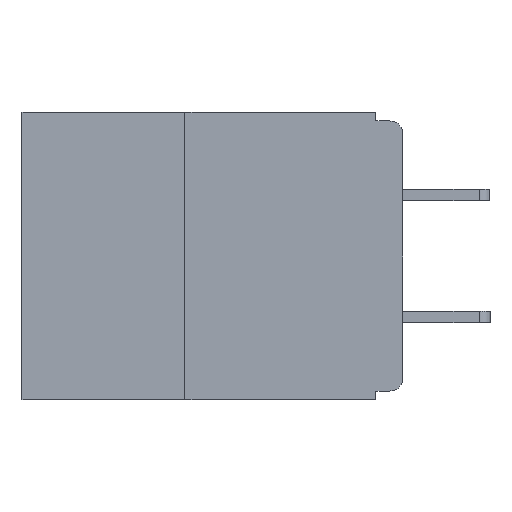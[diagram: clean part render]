
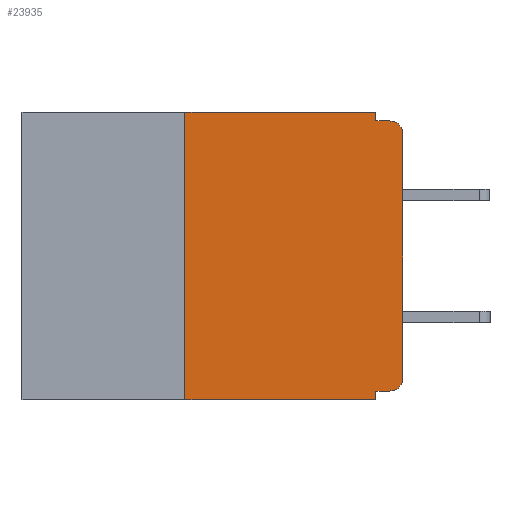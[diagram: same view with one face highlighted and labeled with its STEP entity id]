
A CAD part, left-side view. The second image highlights one B-rep face of the part: STEP entity #23935.
In plain terms, the highlighted planar face has unit normal (-1, 0, 0).
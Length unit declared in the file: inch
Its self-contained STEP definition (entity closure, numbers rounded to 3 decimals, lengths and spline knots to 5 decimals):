
#224 = CARTESIAN_POINT ( 'NONE',  ( 0., 0.031, -0.33 ) ) ;
#714 = EDGE_CURVE ( 'NONE', #23795, #22108, #26850, .T. ) ;
#739 = VECTOR ( 'NONE', #13618, 39.37008 ) ;
#971 = EDGE_LOOP ( 'NONE', ( #21224, #18360, #8289, #6794, #13270, #1096, #14276, #14468, #15029, #21522 ) ) ;
#1096 = ORIENTED_EDGE ( 'NONE', *, *, #19478, .F. ) ;
#1179 = CARTESIAN_POINT ( 'NONE',  ( 0., 0.031, -0.33 ) ) ;
#1496 = VERTEX_POINT ( 'NONE', #224 ) ;
#2697 = LINE ( 'NONE', #28955, #9141 ) ;
#2982 = CARTESIAN_POINT ( 'NONE',  ( 0., 0.031, -0.32 ) ) ;
#3351 = VERTEX_POINT ( 'NONE', #21750 ) ;
#3466 = EDGE_CURVE ( 'NONE', #20962, #15706, #14830, .T. ) ;
#3741 = VECTOR ( 'NONE', #7680, 39.37008 ) ;
#4078 = DIRECTION ( 'NONE',  ( 0., -1., 0. ) ) ;
#5708 = EDGE_CURVE ( 'NONE', #8216, #15706, #6143, .T. ) ;
#6143 = CIRCLE ( 'NONE', #20829, 0.015 ) ;
#6678 = VECTOR ( 'NONE', #13204, 39.37008 ) ;
#6731 = CARTESIAN_POINT ( 'NONE',  ( 0., 0.437, 0. ) ) ;
#6794 = ORIENTED_EDGE ( 'NONE', *, *, #21064, .F. ) ;
#6951 = LINE ( 'NONE', #15800, #11783 ) ;
#7234 = LINE ( 'NONE', #27794, #739 ) ;
#7473 = DIRECTION ( 'NONE',  ( 0., 0., -1. ) ) ;
#7477 = VERTEX_POINT ( 'NONE', #13165 ) ;
#7680 = DIRECTION ( 'NONE',  ( 0., 0., 1. ) ) ;
#7694 = CARTESIAN_POINT ( 'NONE',  ( 0., 0.015, -0.305 ) ) ;
#8216 = VERTEX_POINT ( 'NONE', #28037 ) ;
#8289 = ORIENTED_EDGE ( 'NONE', *, *, #3466, .F. ) ;
#9141 = VECTOR ( 'NONE', #14856, 39.37008 ) ;
#9152 = DIRECTION ( 'NONE',  ( 1., 0., 0. ) ) ;
#10096 = DIRECTION ( 'NONE',  ( 0., 0., -1. ) ) ;
#10869 = VECTOR ( 'NONE', #7473, 39.37008 ) ;
#11783 = VECTOR ( 'NONE', #22987, 39.37008 ) ;
#13165 = CARTESIAN_POINT ( 'NONE',  ( 0., 0.25, -0.33 ) ) ;
#13204 = DIRECTION ( 'NONE',  ( 0., 0., -1. ) ) ;
#13270 = ORIENTED_EDGE ( 'NONE', *, *, #714, .F. ) ;
#13618 = DIRECTION ( 'NONE',  ( 0., 0., 1. ) ) ;
#14276 = ORIENTED_EDGE ( 'NONE', *, *, #16277, .T. ) ;
#14373 = CARTESIAN_POINT ( 'NONE',  ( 0., 0.031, 0. ) ) ;
#14468 = ORIENTED_EDGE ( 'NONE', *, *, #14695, .F. ) ;
#14695 = EDGE_CURVE ( 'NONE', #26090, #1496, #19374, .T. ) ;
#14830 = LINE ( 'NONE', #15309, #26682 ) ;
#14856 = DIRECTION ( 'NONE',  ( 0., 1., 0. ) ) ;
#14902 = CIRCLE ( 'NONE', #28330, 0.015 ) ;
#15029 = ORIENTED_EDGE ( 'NONE', *, *, #18517, .F. ) ;
#15275 = DIRECTION ( 'NONE',  ( 0., -1., 0. ) ) ;
#15309 = CARTESIAN_POINT ( 'NONE',  ( 0., 0., -0.01 ) ) ;
#15706 = VERTEX_POINT ( 'NONE', #28838 ) ;
#15800 = CARTESIAN_POINT ( 'NONE',  ( 0., 0.437, -0.33 ) ) ;
#15920 = FACE_OUTER_BOUND ( 'NONE', #971, .T. ) ;
#16277 = EDGE_CURVE ( 'NONE', #7477, #1496, #6951, .T. ) ;
#18360 = ORIENTED_EDGE ( 'NONE', *, *, #5708, .T. ) ;
#18517 = EDGE_CURVE ( 'NONE', #22694, #26090, #2697, .T. ) ;
#18903 = CARTESIAN_POINT ( 'NONE',  ( 0., 0.437, 0. ) ) ;
#19374 = LINE ( 'NONE', #1179, #6678 ) ;
#19478 = EDGE_CURVE ( 'NONE', #7477, #23795, #7234, .T. ) ;
#19487 = CARTESIAN_POINT ( 'NONE',  ( 0., 0.031, 0. ) ) ;
#20122 = AXIS2_PLACEMENT_3D ( 'NONE', #6731, #9152, #25782 ) ;
#20576 = VECTOR ( 'NONE', #4078, 39.37008 ) ;
#20829 = AXIS2_PLACEMENT_3D ( 'NONE', #27483, #27452, #27343 ) ;
#20962 = VERTEX_POINT ( 'NONE', #28528 ) ;
#21022 = PLANE ( 'NONE',  #20122 ) ;
#21064 = EDGE_CURVE ( 'NONE', #22108, #20962, #23561, .T. ) ;
#21108 = EDGE_CURVE ( 'NONE', #3351, #8216, #28985, .T. ) ;
#21224 = ORIENTED_EDGE ( 'NONE', *, *, #21108, .T. ) ;
#21522 = ORIENTED_EDGE ( 'NONE', *, *, #30047, .T. ) ;
#21750 = CARTESIAN_POINT ( 'NONE',  ( 0., 0., -0.305 ) ) ;
#22108 = VERTEX_POINT ( 'NONE', #14373 ) ;
#22694 = VERTEX_POINT ( 'NONE', #30509 ) ;
#22987 = DIRECTION ( 'NONE',  ( 0., -1., 0. ) ) ;
#23561 = LINE ( 'NONE', #19487, #10869 ) ;
#23795 = VERTEX_POINT ( 'NONE', #29776 ) ;
#23935 = ADVANCED_FACE ( 'NONE', ( #15920 ), #21022, .F. ) ;
#24372 = DIRECTION ( 'NONE',  ( -1., 0., 0. ) ) ;
#25782 = DIRECTION ( 'NONE',  ( 0., 0., -1. ) ) ;
#26090 = VERTEX_POINT ( 'NONE', #2982 ) ;
#26682 = VECTOR ( 'NONE', #15275, 39.37008 ) ;
#26706 = CARTESIAN_POINT ( 'NONE',  ( 0., 0., 0. ) ) ;
#26850 = LINE ( 'NONE', #18903, #20576 ) ;
#27343 = DIRECTION ( 'NONE',  ( 0., 0., -1. ) ) ;
#27452 = DIRECTION ( 'NONE',  ( -1., 0., 0. ) ) ;
#27483 = CARTESIAN_POINT ( 'NONE',  ( 0., 0.015, -0.025 ) ) ;
#27794 = CARTESIAN_POINT ( 'NONE',  ( 0., 0.25, -0.33 ) ) ;
#28037 = CARTESIAN_POINT ( 'NONE',  ( 0., 0., -0.025 ) ) ;
#28330 = AXIS2_PLACEMENT_3D ( 'NONE', #7694, #24372, #10096 ) ;
#28528 = CARTESIAN_POINT ( 'NONE',  ( 0., 0.031, -0.01 ) ) ;
#28838 = CARTESIAN_POINT ( 'NONE',  ( 0., 0.015, -0.01 ) ) ;
#28955 = CARTESIAN_POINT ( 'NONE',  ( 0., 0., -0.32 ) ) ;
#28985 = LINE ( 'NONE', #26706, #3741 ) ;
#29776 = CARTESIAN_POINT ( 'NONE',  ( 0., 0.25, 0. ) ) ;
#30047 = EDGE_CURVE ( 'NONE', #22694, #3351, #14902, .T. ) ;
#30509 = CARTESIAN_POINT ( 'NONE',  ( 0., 0.015, -0.32 ) ) ;
